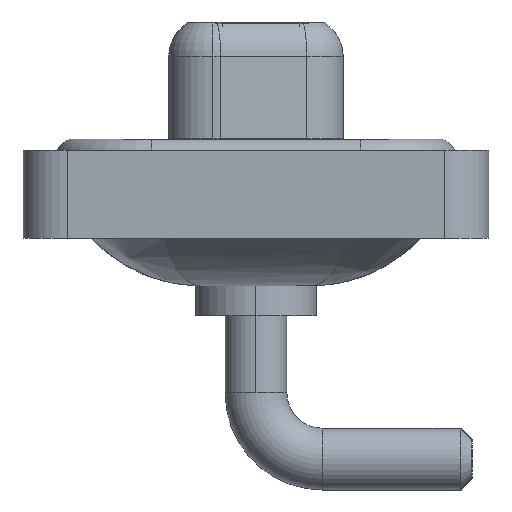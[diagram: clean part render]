
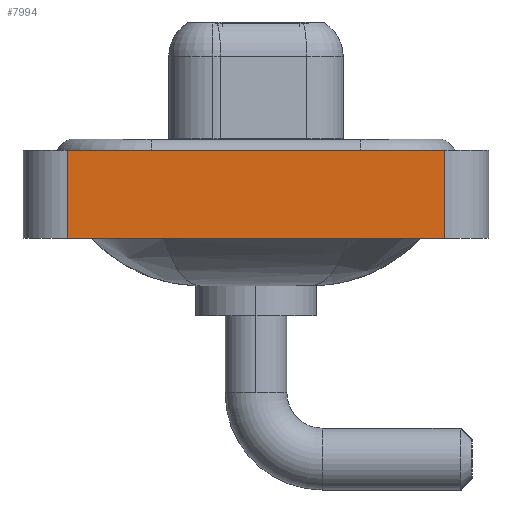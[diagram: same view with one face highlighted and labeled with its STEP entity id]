
A CAD part, left-side view. The second image highlights one B-rep face of the part: STEP entity #7994.
In plain terms, the highlighted planar face has unit normal (-1, 0, 0).
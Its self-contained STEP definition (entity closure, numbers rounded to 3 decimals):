
#410 = EDGE_CURVE ( 'NONE', #3273, #8879, #7277, .T. ) ;
#1288 = LINE ( 'NONE', #9396, #17146 ) ;
#2535 = ORIENTED_EDGE ( 'NONE', *, *, #11302, .F. ) ;
#2924 = CARTESIAN_POINT ( 'NONE',  ( -7.3, 8.55, 0.4 ) ) ;
#2940 = VECTOR ( 'NONE', #7531, 1000. ) ;
#3273 = VERTEX_POINT ( 'NONE', #7129 ) ;
#4540 = CARTESIAN_POINT ( 'NONE',  ( -7.3, -8.55, -3.6 ) ) ;
#5393 = DIRECTION ( 'NONE',  ( -1., 0., 0. ) ) ;
#5657 = CARTESIAN_POINT ( 'NONE',  ( -7.3, -8.55, -3.6 ) ) ;
#6164 = ORIENTED_EDGE ( 'NONE', *, *, #7747, .T. ) ;
#7053 = VERTEX_POINT ( 'NONE', #2924 ) ;
#7129 = CARTESIAN_POINT ( 'NONE',  ( -7.3, -8.55, -3.6 ) ) ;
#7154 = LINE ( 'NONE', #12493, #11053 ) ;
#7277 = LINE ( 'NONE', #4540, #2940 ) ;
#7531 = DIRECTION ( 'NONE',  ( 0., 0., 1. ) ) ;
#7747 = EDGE_CURVE ( 'NONE', #16517, #3273, #1288, .T. ) ;
#7994 = ADVANCED_FACE ( 'NONE', ( #9756 ), #8287, .T. ) ;
#8287 = PLANE ( 'NONE',  #16064 ) ;
#8875 = EDGE_LOOP ( 'NONE', ( #9846, #2535, #14815, #6164 ) ) ;
#8879 = VERTEX_POINT ( 'NONE', #10681 ) ;
#9337 = DIRECTION ( 'NONE',  ( 0., -1., 0. ) ) ;
#9396 = CARTESIAN_POINT ( 'NONE',  ( -7.3, -8.55, -3.6 ) ) ;
#9756 = FACE_OUTER_BOUND ( 'NONE', #8875, .T. ) ;
#9846 = ORIENTED_EDGE ( 'NONE', *, *, #410, .T. ) ;
#10242 = EDGE_CURVE ( 'NONE', #16517, #7053, #7154, .T. ) ;
#10681 = CARTESIAN_POINT ( 'NONE',  ( -7.3, -8.55, 0.4 ) ) ;
#11053 = VECTOR ( 'NONE', #11152, 1000. ) ;
#11152 = DIRECTION ( 'NONE',  ( 0., 0., 1. ) ) ;
#11302 = EDGE_CURVE ( 'NONE', #7053, #8879, #16174, .T. ) ;
#12400 = CARTESIAN_POINT ( 'NONE',  ( -7.3, -8.55, 0.4 ) ) ;
#12493 = CARTESIAN_POINT ( 'NONE',  ( -7.3, 8.55, -3.6 ) ) ;
#14508 = CARTESIAN_POINT ( 'NONE',  ( -7.3, 8.55, -3.6 ) ) ;
#14750 = DIRECTION ( 'NONE',  ( 0., -1., 0. ) ) ;
#14815 = ORIENTED_EDGE ( 'NONE', *, *, #10242, .F. ) ;
#15041 = DIRECTION ( 'NONE',  ( 0., 0., 1. ) ) ;
#15392 = VECTOR ( 'NONE', #9337, 1000. ) ;
#16064 = AXIS2_PLACEMENT_3D ( 'NONE', #5657, #5393, #15041 ) ;
#16174 = LINE ( 'NONE', #12400, #15392 ) ;
#16517 = VERTEX_POINT ( 'NONE', #14508 ) ;
#17146 = VECTOR ( 'NONE', #14750, 1000. ) ;
